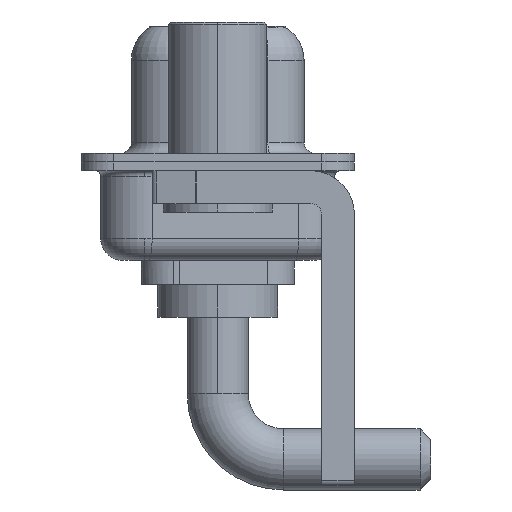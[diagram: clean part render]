
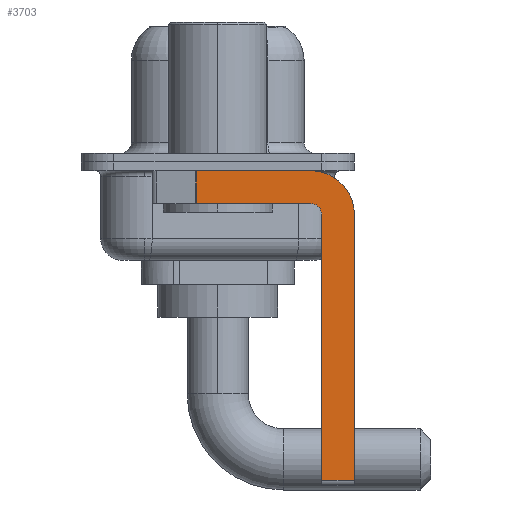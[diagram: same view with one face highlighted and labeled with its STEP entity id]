
A CAD part, left-side view. The second image highlights one B-rep face of the part: STEP entity #3703.
In plain terms, the highlighted planar face has unit normal (-1, 0, 0).
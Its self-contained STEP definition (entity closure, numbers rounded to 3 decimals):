
#515 = CARTESIAN_POINT ( 'NONE',  ( -2.9, 0.978, -1.9 ) ) ;
#597 = VERTEX_POINT ( 'NONE', #6036 ) ;
#600 = CARTESIAN_POINT ( 'NONE',  ( -2.9, -4.25, -14.55 ) ) ;
#657 = EDGE_CURVE ( 'NONE', #6013, #12208, #7781, .T. ) ;
#883 = CARTESIAN_POINT ( 'NONE',  ( -2.9, -4.25, -1.9 ) ) ;
#1001 = AXIS2_PLACEMENT_3D ( 'NONE', #8247, #13044, #7927 ) ;
#1671 = ORIENTED_EDGE ( 'NONE', *, *, #12113, .T. ) ;
#1737 = EDGE_CURVE ( 'NONE', #597, #9463, #7641, .T. ) ;
#1989 = VECTOR ( 'NONE', #9012, 1000. ) ;
#2676 = DIRECTION ( 'NONE',  ( 0., 0., 1. ) ) ;
#3179 = VECTOR ( 'NONE', #11934, 1000. ) ;
#3245 = ORIENTED_EDGE ( 'NONE', *, *, #14732, .F. ) ;
#3281 = EDGE_CURVE ( 'NONE', #597, #8832, #6237, .T. ) ;
#3464 = DIRECTION ( 'NONE',  ( 0., -1., 0. ) ) ;
#3523 = EDGE_CURVE ( 'NONE', #12208, #9382, #6357, .T. ) ;
#3703 = ADVANCED_FACE ( 'NONE', ( #10865 ), #8330, .F. ) ;
#4448 = DIRECTION ( 'NONE',  ( 1., 0., 0. ) ) ;
#4482 = VECTOR ( 'NONE', #11898, 1000. ) ;
#4549 = CARTESIAN_POINT ( 'NONE',  ( -2.9, -6.25, -14.55 ) ) ;
#4697 = VERTEX_POINT ( 'NONE', #5188 ) ;
#4739 = ORIENTED_EDGE ( 'NONE', *, *, #3281, .F. ) ;
#5188 = CARTESIAN_POINT ( 'NONE',  ( -2.9, -6.25, -2.4 ) ) ;
#5824 = CARTESIAN_POINT ( 'NONE',  ( -2.9, -6.25, -2.4 ) ) ;
#6013 = VERTEX_POINT ( 'NONE', #6648 ) ;
#6036 = CARTESIAN_POINT ( 'NONE',  ( -2.9, 0.978, -0.4 ) ) ;
#6235 = VERTEX_POINT ( 'NONE', #4549 ) ;
#6237 = LINE ( 'NONE', #15754, #7132 ) ;
#6305 = ORIENTED_EDGE ( 'NONE', *, *, #12803, .F. ) ;
#6357 = CIRCLE ( 'NONE', #1001, 0.5 ) ;
#6422 = CARTESIAN_POINT ( 'NONE',  ( -2.9, -4.75, -14.8 ) ) ;
#6648 = CARTESIAN_POINT ( 'NONE',  ( -2.9, -4.75, -14.55 ) ) ;
#6900 = AXIS2_PLACEMENT_3D ( 'NONE', #13501, #13276, #15742 ) ;
#7132 = VECTOR ( 'NONE', #3464, 1000. ) ;
#7144 = CARTESIAN_POINT ( 'NONE',  ( -2.9, -4.25, -0.4 ) ) ;
#7551 = ORIENTED_EDGE ( 'NONE', *, *, #1737, .T. ) ;
#7641 = LINE ( 'NONE', #515, #1989 ) ;
#7708 = ORIENTED_EDGE ( 'NONE', *, *, #657, .F. ) ;
#7781 = LINE ( 'NONE', #6422, #8573 ) ;
#7927 = DIRECTION ( 'NONE',  ( 0., 0., 1. ) ) ;
#8247 = CARTESIAN_POINT ( 'NONE',  ( -2.9, -4.25, -2.4 ) ) ;
#8330 = PLANE ( 'NONE',  #6900 ) ;
#8573 = VECTOR ( 'NONE', #2676, 1000. ) ;
#8832 = VERTEX_POINT ( 'NONE', #7144 ) ;
#9012 = DIRECTION ( 'NONE',  ( 0., 0., -1. ) ) ;
#9340 = DIRECTION ( 'NONE',  ( 0., 0., -1. ) ) ;
#9382 = VERTEX_POINT ( 'NONE', #10854 ) ;
#9405 = ORIENTED_EDGE ( 'NONE', *, *, #12971, .F. ) ;
#9463 = VERTEX_POINT ( 'NONE', #9973 ) ;
#9973 = CARTESIAN_POINT ( 'NONE',  ( -2.9, 0.978, -1.9 ) ) ;
#10538 = CARTESIAN_POINT ( 'NONE',  ( -2.9, -4.25, -2.4 ) ) ;
#10854 = CARTESIAN_POINT ( 'NONE',  ( -2.9, -4.25, -1.9 ) ) ;
#10865 = FACE_OUTER_BOUND ( 'NONE', #12287, .T. ) ;
#10877 = ORIENTED_EDGE ( 'NONE', *, *, #3523, .F. ) ;
#11567 = CARTESIAN_POINT ( 'NONE',  ( -2.9, -4.75, -2.4 ) ) ;
#11605 = VECTOR ( 'NONE', #12689, 1000. ) ;
#11731 = LINE ( 'NONE', #600, #11605 ) ;
#11898 = DIRECTION ( 'NONE',  ( 0., 0., -1. ) ) ;
#11934 = DIRECTION ( 'NONE',  ( 0., 1., 0. ) ) ;
#12113 = EDGE_CURVE ( 'NONE', #6013, #6235, #11731, .T. ) ;
#12208 = VERTEX_POINT ( 'NONE', #11567 ) ;
#12287 = EDGE_LOOP ( 'NONE', ( #4739, #7551, #6305, #10877, #7708, #1671, #3245, #9405 ) ) ;
#12689 = DIRECTION ( 'NONE',  ( 0., -1., 0. ) ) ;
#12803 = EDGE_CURVE ( 'NONE', #9382, #9463, #13049, .T. ) ;
#12971 = EDGE_CURVE ( 'NONE', #8832, #4697, #14898, .T. ) ;
#13044 = DIRECTION ( 'NONE',  ( -1., 0., 0. ) ) ;
#13049 = LINE ( 'NONE', #883, #3179 ) ;
#13276 = DIRECTION ( 'NONE',  ( 1., 0., 0. ) ) ;
#13501 = CARTESIAN_POINT ( 'NONE',  ( -2.9, -4.25, -2.4 ) ) ;
#14511 = LINE ( 'NONE', #5824, #4482 ) ;
#14732 = EDGE_CURVE ( 'NONE', #4697, #6235, #14511, .T. ) ;
#14898 = CIRCLE ( 'NONE', #15159, 2. ) ;
#15159 = AXIS2_PLACEMENT_3D ( 'NONE', #10538, #4448, #9340 ) ;
#15742 = DIRECTION ( 'NONE',  ( 0., 0., -1. ) ) ;
#15754 = CARTESIAN_POINT ( 'NONE',  ( -2.9, 3., -0.4 ) ) ;
